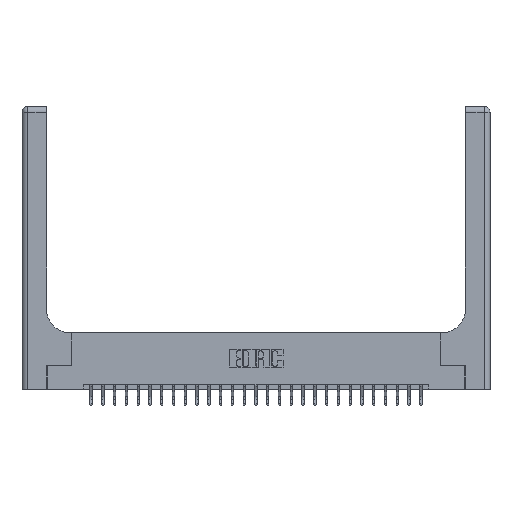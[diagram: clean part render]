
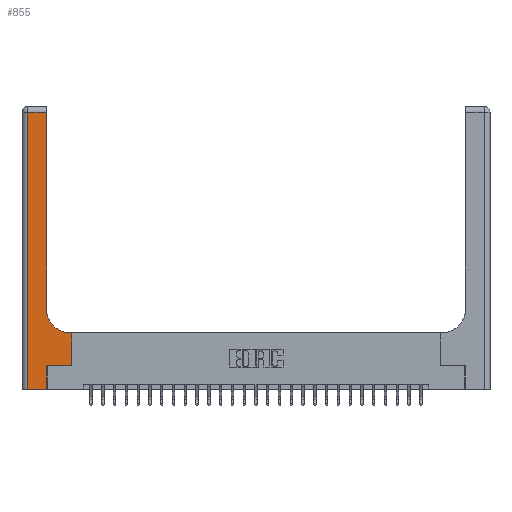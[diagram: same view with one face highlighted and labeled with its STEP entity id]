
A CAD part, top view. The second image highlights one B-rep face of the part: STEP entity #855.
In plain terms, the highlighted planar face has unit normal (0, 0, 1).
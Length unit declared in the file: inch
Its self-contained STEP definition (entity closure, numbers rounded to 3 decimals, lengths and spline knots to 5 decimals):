
#739 = ORIENTED_EDGE ( 'NONE', *, *, #7387, .T. ) ;
#751 = VERTEX_POINT ( 'NONE', #10089 ) ;
#855 = ADVANCED_FACE ( 'NONE', ( #19701 ), #6713, .F. ) ;
#878 = ORIENTED_EDGE ( 'NONE', *, *, #22905, .T. ) ;
#1379 = CARTESIAN_POINT ( 'NONE',  ( 0.26, 3., 0.37 ) ) ;
#1570 = CARTESIAN_POINT ( 'NONE',  ( 0.26, 0.85, 0.37 ) ) ;
#1702 = DIRECTION ( 'NONE',  ( 0., -1., 0. ) ) ;
#1791 = CARTESIAN_POINT ( 'NONE',  ( 0.26, 0.6, 0.37 ) ) ;
#1913 = EDGE_CURVE ( 'NONE', #9862, #10114, #25841, .T. ) ;
#2262 = CARTESIAN_POINT ( 'NONE',  ( 0.265, 0.25, 0.37 ) ) ;
#2639 = CARTESIAN_POINT ( 'NONE',  ( 0.06, 2.94, 0.37 ) ) ;
#3715 = CARTESIAN_POINT ( 'NONE',  ( 0., 2.94, 0.37 ) ) ;
#4394 = EDGE_LOOP ( 'NONE', ( #20143, #19270, #18610, #878, #16193, #12826, #22215, #739, #11597 ) ) ;
#4692 = CARTESIAN_POINT ( 'NONE',  ( 0., 0., 0.37 ) ) ;
#4706 = DIRECTION ( 'NONE',  ( 0., 0., -1. ) ) ;
#4843 = CARTESIAN_POINT ( 'NONE',  ( 0.528, 0.25, 0.37 ) ) ;
#4990 = VERTEX_POINT ( 'NONE', #16392 ) ;
#5034 = CIRCLE ( 'NONE', #24348, 0.25 ) ;
#5313 = CARTESIAN_POINT ( 'NONE',  ( 0.528, 0.25, 0.37 ) ) ;
#5588 = VERTEX_POINT ( 'NONE', #2262 ) ;
#5751 = VECTOR ( 'NONE', #23805, 39.37008 ) ;
#5997 = VECTOR ( 'NONE', #21670, 39.37008 ) ;
#6179 = EDGE_CURVE ( 'NONE', #4990, #5588, #7531, .T. ) ;
#6566 = VECTOR ( 'NONE', #13658, 39.37008 ) ;
#6713 = PLANE ( 'NONE',  #9191 ) ;
#7221 = CARTESIAN_POINT ( 'NONE',  ( 0.51, 0.85, 0.37 ) ) ;
#7386 = CARTESIAN_POINT ( 'NONE',  ( 0.06, 0., 0.37 ) ) ;
#7387 = EDGE_CURVE ( 'NONE', #25231, #751, #7548, .T. ) ;
#7531 = LINE ( 'NONE', #15746, #5997 ) ;
#7548 = LINE ( 'NONE', #1791, #18906 ) ;
#7599 = VECTOR ( 'NONE', #1702, 39.37008 ) ;
#9191 = AXIS2_PLACEMENT_3D ( 'NONE', #13167, #4706, #11019 ) ;
#9822 = EDGE_CURVE ( 'NONE', #10114, #14951, #13399, .T. ) ;
#9862 = VERTEX_POINT ( 'NONE', #1570 ) ;
#10089 = CARTESIAN_POINT ( 'NONE',  ( 0.51, 0.6, 0.37 ) ) ;
#10114 = VERTEX_POINT ( 'NONE', #18756 ) ;
#10509 = VERTEX_POINT ( 'NONE', #4843 ) ;
#10560 = CARTESIAN_POINT ( 'NONE',  ( 0.528, 0.6, 0.37 ) ) ;
#10921 = VECTOR ( 'NONE', #21704, 39.37008 ) ;
#11019 = DIRECTION ( 'NONE',  ( -1., 0., 0. ) ) ;
#11597 = ORIENTED_EDGE ( 'NONE', *, *, #23095, .T. ) ;
#11600 = DIRECTION ( 'NONE',  ( -1., 0., 0. ) ) ;
#11738 = EDGE_CURVE ( 'NONE', #5588, #10509, #26065, .T. ) ;
#12826 = ORIENTED_EDGE ( 'NONE', *, *, #11738, .T. ) ;
#13167 = CARTESIAN_POINT ( 'NONE',  ( 0., 3., 0.37 ) ) ;
#13399 = LINE ( 'NONE', #3715, #6566 ) ;
#13553 = CARTESIAN_POINT ( 'NONE',  ( 0.265, 0.25, 0.37 ) ) ;
#13658 = DIRECTION ( 'NONE',  ( -1., 0., 0. ) ) ;
#13670 = DIRECTION ( 'NONE',  ( 1., 0., 0. ) ) ;
#13973 = EDGE_CURVE ( 'NONE', #10509, #25231, #17536, .T. ) ;
#14022 = VECTOR ( 'NONE', #18664, 39.37008 ) ;
#14951 = VERTEX_POINT ( 'NONE', #2639 ) ;
#15746 = CARTESIAN_POINT ( 'NONE',  ( 0.265, 0., 0.37 ) ) ;
#16063 = CARTESIAN_POINT ( 'NONE',  ( 0.06, 3., 0.37 ) ) ;
#16193 = ORIENTED_EDGE ( 'NONE', *, *, #6179, .T. ) ;
#16392 = CARTESIAN_POINT ( 'NONE',  ( 0.265, 0., 0.37 ) ) ;
#17536 = LINE ( 'NONE', #5313, #10921 ) ;
#18610 = ORIENTED_EDGE ( 'NONE', *, *, #23865, .T. ) ;
#18664 = DIRECTION ( 'NONE',  ( 1., 0., 0. ) ) ;
#18756 = CARTESIAN_POINT ( 'NONE',  ( 0.26, 2.94, 0.37 ) ) ;
#18906 = VECTOR ( 'NONE', #11600, 39.37008 ) ;
#19270 = ORIENTED_EDGE ( 'NONE', *, *, #9822, .T. ) ;
#19701 = FACE_OUTER_BOUND ( 'NONE', #4394, .T. ) ;
#20143 = ORIENTED_EDGE ( 'NONE', *, *, #1913, .T. ) ;
#20272 = VECTOR ( 'NONE', #21760, 39.37008 ) ;
#20677 = LINE ( 'NONE', #4692, #14022 ) ;
#21670 = DIRECTION ( 'NONE',  ( 0., 1., 0. ) ) ;
#21704 = DIRECTION ( 'NONE',  ( 0., 1., 0. ) ) ;
#21760 = DIRECTION ( 'NONE',  ( 1., 0., 0. ) ) ;
#22215 = ORIENTED_EDGE ( 'NONE', *, *, #13973, .T. ) ;
#22521 = VERTEX_POINT ( 'NONE', #7386 ) ;
#22905 = EDGE_CURVE ( 'NONE', #22521, #4990, #20677, .T. ) ;
#23095 = EDGE_CURVE ( 'NONE', #751, #9862, #5034, .T. ) ;
#23624 = DIRECTION ( 'NONE',  ( 0., 0., -1. ) ) ;
#23805 = DIRECTION ( 'NONE',  ( 0., 1., 0. ) ) ;
#23865 = EDGE_CURVE ( 'NONE', #14951, #22521, #26292, .T. ) ;
#24348 = AXIS2_PLACEMENT_3D ( 'NONE', #7221, #23624, #13670 ) ;
#25231 = VERTEX_POINT ( 'NONE', #10560 ) ;
#25841 = LINE ( 'NONE', #1379, #5751 ) ;
#26065 = LINE ( 'NONE', #13553, #20272 ) ;
#26292 = LINE ( 'NONE', #16063, #7599 ) ;
